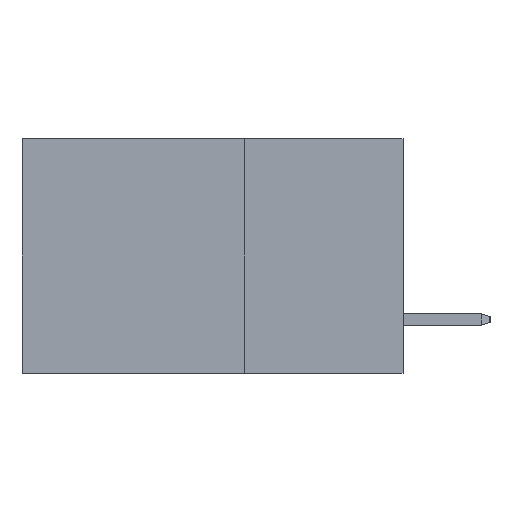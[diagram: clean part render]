
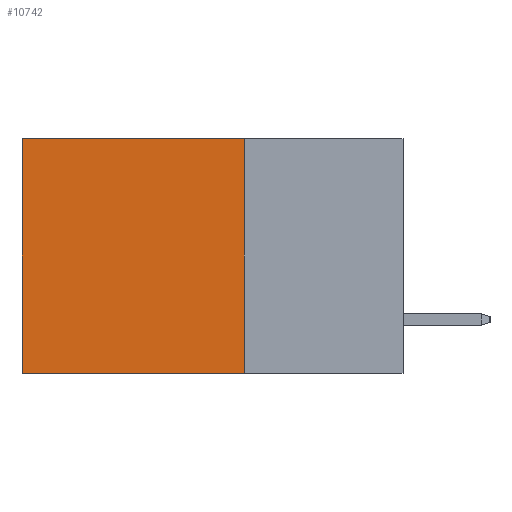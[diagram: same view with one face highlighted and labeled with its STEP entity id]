
A CAD part, left-side view. The second image highlights one B-rep face of the part: STEP entity #10742.
In plain terms, the highlighted planar face has unit normal (-1, 0, 0).
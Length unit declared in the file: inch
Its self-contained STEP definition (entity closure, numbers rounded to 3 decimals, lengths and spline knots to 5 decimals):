
#4 = VECTOR ( 'NONE', #1726, 39.37008 ) ;
#11 = ORIENTED_EDGE ( 'NONE', *, *, #742, .F. ) ;
#35 = ORIENTED_EDGE ( 'NONE', *, *, #9429, .T. ) ;
#48 = AXIS2_PLACEMENT_3D ( 'NONE', #7834, #157, #2007 ) ;
#156 = EDGE_CURVE ( 'NONE', #628, #6846, #8461, .T. ) ;
#157 = DIRECTION ( 'NONE',  ( 1., 0., 0. ) ) ;
#279 = CARTESIAN_POINT ( 'NONE',  ( 0.2875, 0.25, -0.37 ) ) ;
#628 = VERTEX_POINT ( 'NONE', #9451 ) ;
#742 = EDGE_CURVE ( 'NONE', #6846, #12124, #8283, .T. ) ;
#911 = ORIENTED_EDGE ( 'NONE', *, *, #156, .F. ) ;
#1102 = PLANE ( 'NONE',  #48 ) ;
#1726 = DIRECTION ( 'NONE',  ( 0., 0., -1. ) ) ;
#2007 = DIRECTION ( 'NONE',  ( 0., 0., -1. ) ) ;
#2043 = CARTESIAN_POINT ( 'NONE',  ( 0.2875, 0.25, 0. ) ) ;
#2504 = VECTOR ( 'NONE', #8545, 39.37008 ) ;
#2852 = DIRECTION ( 'NONE',  ( 0., 1., 0. ) ) ;
#3045 = FACE_OUTER_BOUND ( 'NONE', #5733, .T. ) ;
#3406 = CARTESIAN_POINT ( 'NONE',  ( 0.2875, 0.6, 0. ) ) ;
#3842 = VECTOR ( 'NONE', #2852, 39.37008 ) ;
#4125 = DIRECTION ( 'NONE',  ( 0., 1., 0. ) ) ;
#4521 = LINE ( 'NONE', #6565, #2504 ) ;
#4744 = VERTEX_POINT ( 'NONE', #3406 ) ;
#5092 = VECTOR ( 'NONE', #4125, 39.37008 ) ;
#5733 = EDGE_LOOP ( 'NONE', ( #35, #11, #911, #9183 ) ) ;
#6413 = CARTESIAN_POINT ( 'NONE',  ( 0.2875, 0.25, 0. ) ) ;
#6565 = CARTESIAN_POINT ( 'NONE',  ( 0.2875, 0.6, 0. ) ) ;
#6846 = VERTEX_POINT ( 'NONE', #7134 ) ;
#7134 = CARTESIAN_POINT ( 'NONE',  ( 0.2875, 0.25, -0.37 ) ) ;
#7834 = CARTESIAN_POINT ( 'NONE',  ( 0.2875, 0.25, 0. ) ) ;
#8283 = LINE ( 'NONE', #279, #5092 ) ;
#8461 = LINE ( 'NONE', #6413, #4 ) ;
#8545 = DIRECTION ( 'NONE',  ( 0., 0., -1. ) ) ;
#8725 = LINE ( 'NONE', #2043, #3842 ) ;
#9183 = ORIENTED_EDGE ( 'NONE', *, *, #12032, .T. ) ;
#9429 = EDGE_CURVE ( 'NONE', #4744, #12124, #4521, .T. ) ;
#9451 = CARTESIAN_POINT ( 'NONE',  ( 0.2875, 0.25, 0. ) ) ;
#10742 = ADVANCED_FACE ( 'NONE', ( #3045 ), #1102, .F. ) ;
#11750 = CARTESIAN_POINT ( 'NONE',  ( 0.2875, 0.6, -0.37 ) ) ;
#12032 = EDGE_CURVE ( 'NONE', #628, #4744, #8725, .T. ) ;
#12124 = VERTEX_POINT ( 'NONE', #11750 ) ;
